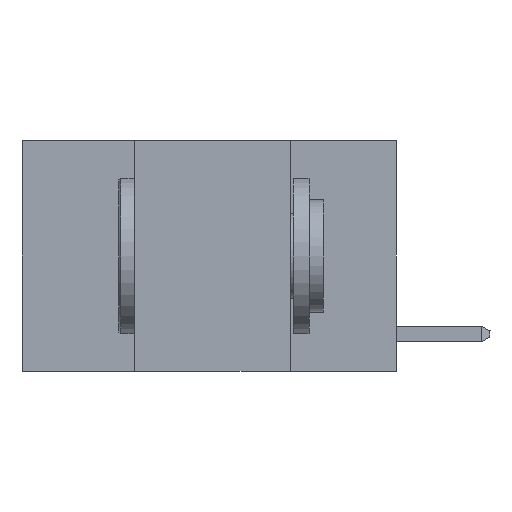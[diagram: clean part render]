
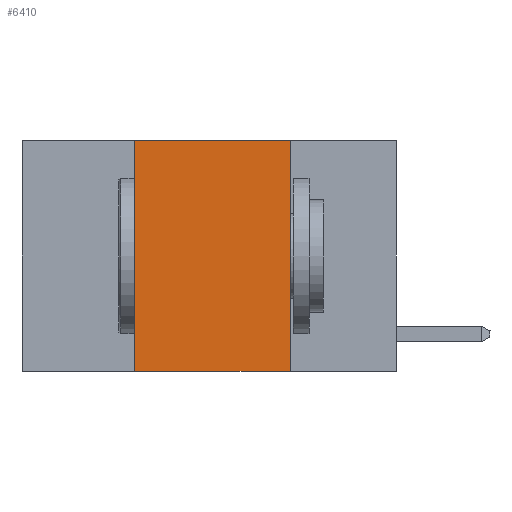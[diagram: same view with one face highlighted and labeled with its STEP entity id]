
A CAD part, left-side view. The second image highlights one B-rep face of the part: STEP entity #6410.
In plain terms, the highlighted planar face has unit normal (-1, 0, 0).
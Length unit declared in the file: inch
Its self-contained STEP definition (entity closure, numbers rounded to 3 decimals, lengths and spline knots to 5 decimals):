
#732 = VERTEX_POINT ( 'NONE', #2505 ) ;
#1503 = FACE_OUTER_BOUND ( 'NONE', #16059, .T. ) ;
#1672 = VERTEX_POINT ( 'NONE', #14110 ) ;
#2505 = CARTESIAN_POINT ( 'NONE',  ( 0., 0.17, 0. ) ) ;
#2585 = EDGE_CURVE ( 'NONE', #6767, #1672, #17456, .T. ) ;
#2592 = VECTOR ( 'NONE', #10383, 39.37008 ) ;
#3028 = PLANE ( 'NONE',  #12147 ) ;
#3192 = ORIENTED_EDGE ( 'NONE', *, *, #14572, .F. ) ;
#4327 = LINE ( 'NONE', #9137, #15050 ) ;
#4456 = DIRECTION ( 'NONE',  ( 0., 0., -1. ) ) ;
#4734 = DIRECTION ( 'NONE',  ( 0., 0., 1. ) ) ;
#5316 = ORIENTED_EDGE ( 'NONE', *, *, #2585, .F. ) ;
#5451 = CARTESIAN_POINT ( 'NONE',  ( 0., 0.17, -0.37 ) ) ;
#5802 = CARTESIAN_POINT ( 'NONE',  ( 0., 0.6, 0. ) ) ;
#6392 = VECTOR ( 'NONE', #4734, 39.37008 ) ;
#6410 = ADVANCED_FACE ( 'NONE', ( #1503 ), #3028, .F. ) ;
#6767 = VERTEX_POINT ( 'NONE', #13552 ) ;
#8980 = CARTESIAN_POINT ( 'NONE',  ( 0., 0.6, 0. ) ) ;
#9137 = CARTESIAN_POINT ( 'NONE',  ( 0., 0.17, 0. ) ) ;
#10032 = VECTOR ( 'NONE', #16014, 39.37008 ) ;
#10154 = LINE ( 'NONE', #8980, #2592 ) ;
#10301 = ORIENTED_EDGE ( 'NONE', *, *, #15359, .F. ) ;
#10383 = DIRECTION ( 'NONE',  ( 0., -1., 0. ) ) ;
#10396 = CARTESIAN_POINT ( 'NONE',  ( 0., 0.42, 0. ) ) ;
#11460 = EDGE_CURVE ( 'NONE', #6767, #14913, #17702, .T. ) ;
#12147 = AXIS2_PLACEMENT_3D ( 'NONE', #5802, #12894, #4456 ) ;
#12894 = DIRECTION ( 'NONE',  ( 1., 0., 0. ) ) ;
#13111 = ORIENTED_EDGE ( 'NONE', *, *, #11460, .T. ) ;
#13552 = CARTESIAN_POINT ( 'NONE',  ( 0., 0.42, -0.37 ) ) ;
#14110 = CARTESIAN_POINT ( 'NONE',  ( 0., 0.42, 0. ) ) ;
#14572 = EDGE_CURVE ( 'NONE', #1672, #732, #10154, .T. ) ;
#14692 = CARTESIAN_POINT ( 'NONE',  ( 0., 0.6, -0.37 ) ) ;
#14913 = VERTEX_POINT ( 'NONE', #5451 ) ;
#15050 = VECTOR ( 'NONE', #16068, 39.37008 ) ;
#15359 = EDGE_CURVE ( 'NONE', #732, #14913, #4327, .T. ) ;
#16014 = DIRECTION ( 'NONE',  ( 0., -1., 0. ) ) ;
#16059 = EDGE_LOOP ( 'NONE', ( #10301, #3192, #5316, #13111 ) ) ;
#16068 = DIRECTION ( 'NONE',  ( 0., 0., -1. ) ) ;
#17456 = LINE ( 'NONE', #10396, #6392 ) ;
#17702 = LINE ( 'NONE', #14692, #10032 ) ;
